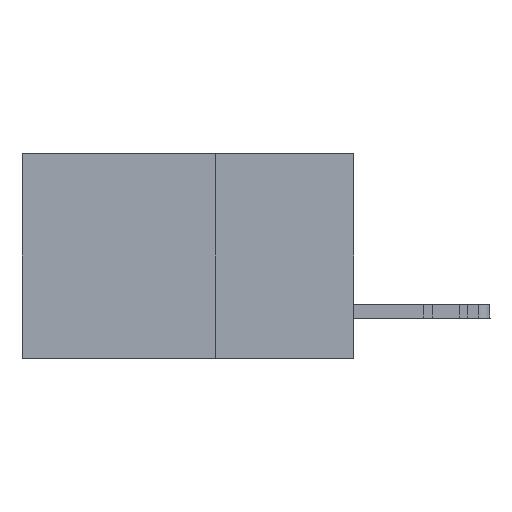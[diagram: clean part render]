
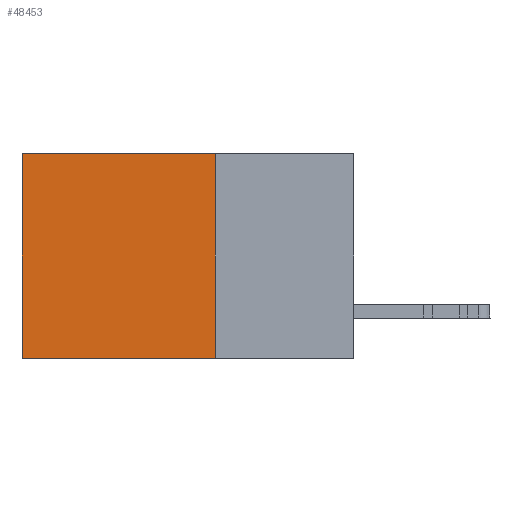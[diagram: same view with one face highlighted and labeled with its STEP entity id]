
A CAD part, left-side view. The second image highlights one B-rep face of the part: STEP entity #48453.
In plain terms, the highlighted planar face has unit normal (-1, 0, 0).
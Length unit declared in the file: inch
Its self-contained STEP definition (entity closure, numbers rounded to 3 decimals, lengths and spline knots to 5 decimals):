
#106 = DIRECTION ( 'NONE',  ( 0., 0., -1. ) ) ;
#1613 = CARTESIAN_POINT ( 'NONE',  ( 0.2875, 0.6, 0. ) ) ;
#1842 = FACE_OUTER_BOUND ( 'NONE', #44033, .T. ) ;
#2998 = DIRECTION ( 'NONE',  ( 0., 0., -1. ) ) ;
#6432 = VECTOR ( 'NONE', #34563, 39.37008 ) ;
#6561 = DIRECTION ( 'NONE',  ( 0., 1., 0. ) ) ;
#6795 = CARTESIAN_POINT ( 'NONE',  ( 0.2875, 0.6, 0. ) ) ;
#9437 = ORIENTED_EDGE ( 'NONE', *, *, #36010, .F. ) ;
#12068 = CARTESIAN_POINT ( 'NONE',  ( 0.2875, 0.25, 0. ) ) ;
#12620 = ORIENTED_EDGE ( 'NONE', *, *, #48685, .T. ) ;
#13097 = DIRECTION ( 'NONE',  ( 0., 0., -1. ) ) ;
#14064 = VERTEX_POINT ( 'NONE', #6795 ) ;
#15423 = ORIENTED_EDGE ( 'NONE', *, *, #41174, .F. ) ;
#16128 = ORIENTED_EDGE ( 'NONE', *, *, #19200, .T. ) ;
#16381 = LINE ( 'NONE', #50281, #6432 ) ;
#17314 = LINE ( 'NONE', #1613, #23488 ) ;
#19200 = EDGE_CURVE ( 'NONE', #20827, #14064, #33603, .T. ) ;
#19398 = CARTESIAN_POINT ( 'NONE',  ( 0.2875, 0.25, 0. ) ) ;
#20827 = VERTEX_POINT ( 'NONE', #35847 ) ;
#23488 = VECTOR ( 'NONE', #13097, 39.37008 ) ;
#33603 = LINE ( 'NONE', #19398, #42849 ) ;
#34205 = LINE ( 'NONE', #46387, #43453 ) ;
#34213 = CARTESIAN_POINT ( 'NONE',  ( 0.2875, 0.25, -0.37 ) ) ;
#34563 = DIRECTION ( 'NONE',  ( 0., 1., 0. ) ) ;
#35847 = CARTESIAN_POINT ( 'NONE',  ( 0.2875, 0.25, 0. ) ) ;
#36010 = EDGE_CURVE ( 'NONE', #20827, #44535, #34205, .T. ) ;
#36092 = PLANE ( 'NONE',  #39598 ) ;
#38235 = CARTESIAN_POINT ( 'NONE',  ( 0.2875, 0.6, -0.37 ) ) ;
#39598 = AXIS2_PLACEMENT_3D ( 'NONE', #12068, #48142, #106 ) ;
#41174 = EDGE_CURVE ( 'NONE', #44535, #47659, #16381, .T. ) ;
#42849 = VECTOR ( 'NONE', #6561, 39.37008 ) ;
#43453 = VECTOR ( 'NONE', #2998, 39.37008 ) ;
#44033 = EDGE_LOOP ( 'NONE', ( #12620, #15423, #9437, #16128 ) ) ;
#44535 = VERTEX_POINT ( 'NONE', #34213 ) ;
#46387 = CARTESIAN_POINT ( 'NONE',  ( 0.2875, 0.25, 0. ) ) ;
#47659 = VERTEX_POINT ( 'NONE', #38235 ) ;
#48142 = DIRECTION ( 'NONE',  ( 1., 0., 0. ) ) ;
#48453 = ADVANCED_FACE ( 'NONE', ( #1842 ), #36092, .F. ) ;
#48685 = EDGE_CURVE ( 'NONE', #14064, #47659, #17314, .T. ) ;
#50281 = CARTESIAN_POINT ( 'NONE',  ( 0.2875, 0.25, -0.37 ) ) ;
